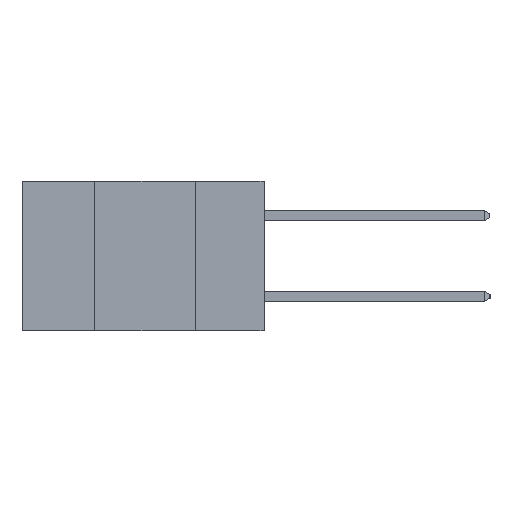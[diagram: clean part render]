
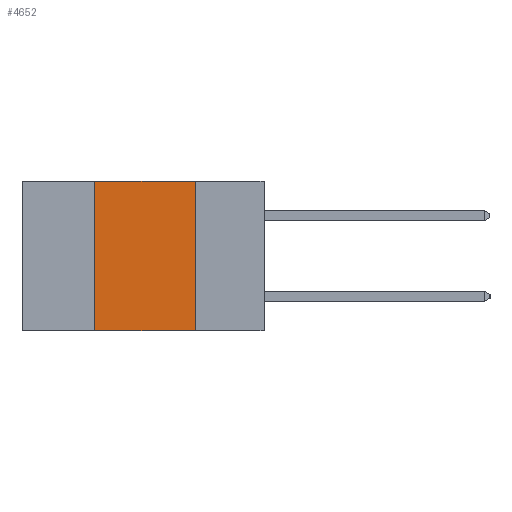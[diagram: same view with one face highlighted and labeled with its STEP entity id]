
A CAD part, left-side view. The second image highlights one B-rep face of the part: STEP entity #4652.
In plain terms, the highlighted planar face has unit normal (-1, 0, 0).
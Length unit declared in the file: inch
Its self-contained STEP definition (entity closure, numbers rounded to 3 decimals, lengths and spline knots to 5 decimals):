
#48 = LINE ( 'NONE', #10206, #9225 ) ;
#124 = LINE ( 'NONE', #1693, #4950 ) ;
#245 = ORIENTED_EDGE ( 'NONE', *, *, #9106, .F. ) ;
#301 = CARTESIAN_POINT ( 'NONE',  ( 0., 0.17, -0.37 ) ) ;
#705 = ORIENTED_EDGE ( 'NONE', *, *, #4763, .T. ) ;
#782 = LINE ( 'NONE', #301, #9824 ) ;
#933 = AXIS2_PLACEMENT_3D ( 'NONE', #3090, #3072, #3031 ) ;
#1067 = FACE_OUTER_BOUND ( 'NONE', #9036, .T. ) ;
#1084 = CARTESIAN_POINT ( 'NONE',  ( 0., 0.17, -0.37 ) ) ;
#1132 = CARTESIAN_POINT ( 'NONE',  ( 0., 0.42, 0. ) ) ;
#1658 = DIRECTION ( 'NONE',  ( 0., -1., 0. ) ) ;
#1693 = CARTESIAN_POINT ( 'NONE',  ( 0., 0.6, -0.37 ) ) ;
#1849 = EDGE_CURVE ( 'NONE', #4234, #8708, #782, .T. ) ;
#3031 = DIRECTION ( 'NONE',  ( 0., 0., -1. ) ) ;
#3072 = DIRECTION ( 'NONE',  ( 1., 0., 0. ) ) ;
#3090 = CARTESIAN_POINT ( 'NONE',  ( 0., 0.6, 0. ) ) ;
#3273 = PLANE ( 'NONE',  #933 ) ;
#4090 = DIRECTION ( 'NONE',  ( 0., 0., -1. ) ) ;
#4234 = VERTEX_POINT ( 'NONE', #10489 ) ;
#4652 = ADVANCED_FACE ( 'NONE', ( #1067 ), #3273, .F. ) ;
#4763 = EDGE_CURVE ( 'NONE', #10467, #8708, #124, .T. ) ;
#4950 = VECTOR ( 'NONE', #1658, 39.37008 ) ;
#4968 = DIRECTION ( 'NONE',  ( 0., 0., 1. ) ) ;
#5105 = DIRECTION ( 'NONE',  ( 0., -1., 0. ) ) ;
#7263 = CARTESIAN_POINT ( 'NONE',  ( 0., 0.42, -0.37 ) ) ;
#7523 = EDGE_CURVE ( 'NONE', #10467, #8762, #10573, .T. ) ;
#7573 = CARTESIAN_POINT ( 'NONE',  ( 0., 0.42, -0.37 ) ) ;
#8432 = VECTOR ( 'NONE', #4968, 39.37008 ) ;
#8708 = VERTEX_POINT ( 'NONE', #1084 ) ;
#8762 = VERTEX_POINT ( 'NONE', #1132 ) ;
#9036 = EDGE_LOOP ( 'NONE', ( #9642, #245, #9117, #705 ) ) ;
#9106 = EDGE_CURVE ( 'NONE', #8762, #4234, #48, .T. ) ;
#9117 = ORIENTED_EDGE ( 'NONE', *, *, #7523, .F. ) ;
#9225 = VECTOR ( 'NONE', #5105, 39.37008 ) ;
#9642 = ORIENTED_EDGE ( 'NONE', *, *, #1849, .F. ) ;
#9824 = VECTOR ( 'NONE', #4090, 39.37008 ) ;
#10206 = CARTESIAN_POINT ( 'NONE',  ( 0., 0.6, 0. ) ) ;
#10467 = VERTEX_POINT ( 'NONE', #7263 ) ;
#10489 = CARTESIAN_POINT ( 'NONE',  ( 0., 0.17, 0. ) ) ;
#10573 = LINE ( 'NONE', #7573, #8432 ) ;
